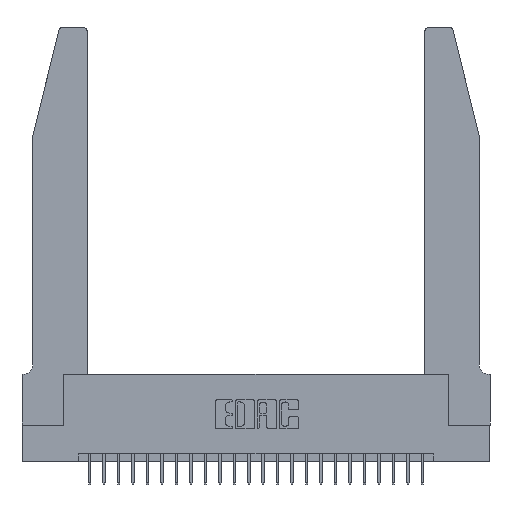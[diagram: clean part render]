
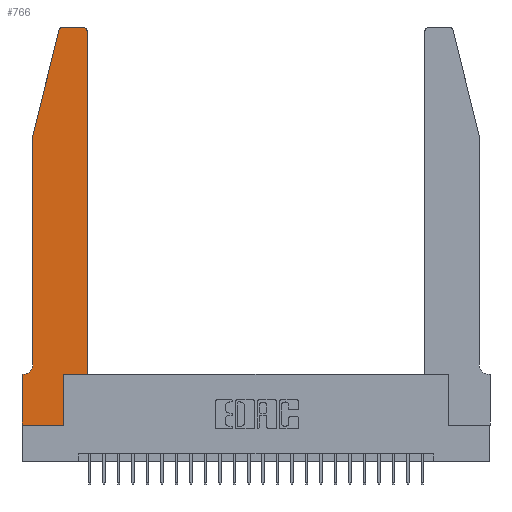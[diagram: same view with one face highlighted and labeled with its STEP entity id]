
A CAD part, top view. The second image highlights one B-rep face of the part: STEP entity #766.
In plain terms, the highlighted planar face has unit normal (0, 0, 1).
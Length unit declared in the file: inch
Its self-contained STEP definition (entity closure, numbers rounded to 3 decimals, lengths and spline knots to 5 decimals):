
#154 = CARTESIAN_POINT ( 'NONE',  ( 0.4505, 0.35, 0.37 ) ) ;
#517 = LINE ( 'NONE', #7419, #10268 ) ;
#766 = ADVANCED_FACE ( 'NONE', ( #21675 ), #9268, .T. ) ;
#827 = EDGE_CURVE ( 'NONE', #11715, #16014, #4376, .T. ) ;
#1599 = VERTEX_POINT ( 'NONE', #9152 ) ;
#2310 = DIRECTION ( 'NONE',  ( 0., 1., 0. ) ) ;
#3278 = EDGE_CURVE ( 'NONE', #14637, #11715, #20070, .T. ) ;
#4025 = CARTESIAN_POINT ( 'NONE',  ( 0., 0., 0.37 ) ) ;
#4050 = VECTOR ( 'NONE', #2310, 39.37008 ) ;
#4246 = ORIENTED_EDGE ( 'NONE', *, *, #5903, .T. ) ;
#4376 = LINE ( 'NONE', #4025, #19805 ) ;
#4411 = EDGE_CURVE ( 'NONE', #21281, #14637, #6228, .T. ) ;
#4421 = ORIENTED_EDGE ( 'NONE', *, *, #7641, .T. ) ;
#4755 = LINE ( 'NONE', #24394, #8960 ) ;
#4835 = CARTESIAN_POINT ( 'NONE',  ( 0.0055, 0.35, 0.37 ) ) ;
#4850 = CARTESIAN_POINT ( 'NONE',  ( 0.0755, 0.35, 0.37 ) ) ;
#4903 = VECTOR ( 'NONE', #20922, 39.37008 ) ;
#5070 = CARTESIAN_POINT ( 'NONE',  ( 0.0755, 2., 0.37 ) ) ;
#5484 = CARTESIAN_POINT ( 'NONE',  ( 0.2865, 0., 0.37 ) ) ;
#5593 = ORIENTED_EDGE ( 'NONE', *, *, #4411, .T. ) ;
#5618 = DIRECTION ( 'NONE',  ( 0., -1., 0. ) ) ;
#5797 = DIRECTION ( 'NONE',  ( 1., 0., 0. ) ) ;
#5903 = EDGE_CURVE ( 'NONE', #15294, #24518, #16241, .T. ) ;
#6228 = LINE ( 'NONE', #4850, #4903 ) ;
#6866 = LINE ( 'NONE', #19316, #15716 ) ;
#6924 = CARTESIAN_POINT ( 'NONE',  ( 0.2865, 0.35, 0.37 ) ) ;
#7098 = ORIENTED_EDGE ( 'NONE', *, *, #3278, .T. ) ;
#7419 = CARTESIAN_POINT ( 'NONE',  ( 0.2865, 0.35, 0.37 ) ) ;
#7463 = CARTESIAN_POINT ( 'NONE',  ( 0.2605, 2.75, 0.37 ) ) ;
#7641 = EDGE_CURVE ( 'NONE', #16014, #21268, #517, .T. ) ;
#7769 = VECTOR ( 'NONE', #21515, 39.37008 ) ;
#8455 = CARTESIAN_POINT ( 'NONE',  ( 0.0055, 0.42, 0.37 ) ) ;
#8582 = CARTESIAN_POINT ( 'NONE',  ( 0.4205, 2.72, 0.37 ) ) ;
#8960 = VECTOR ( 'NONE', #12621, 39.37008 ) ;
#9152 = CARTESIAN_POINT ( 'NONE',  ( 0.4205, 2.75, 0.37 ) ) ;
#9268 = PLANE ( 'NONE',  #25389 ) ;
#9486 = VECTOR ( 'NONE', #16763, 39.37008 ) ;
#9494 = ORIENTED_EDGE ( 'NONE', *, *, #16354, .T. ) ;
#9497 = CARTESIAN_POINT ( 'NONE',  ( 0., 0.35, 0.37 ) ) ;
#10060 = DIRECTION ( 'NONE',  ( 0., 0., 1. ) ) ;
#10237 = DIRECTION ( 'NONE',  ( 1., 0., 0. ) ) ;
#10268 = VECTOR ( 'NONE', #21390, 39.37008 ) ;
#10269 = DIRECTION ( 'NONE',  ( 0., 0., 1. ) ) ;
#10503 = DIRECTION ( 'NONE',  ( -1., 0., 0. ) ) ;
#10630 = DIRECTION ( 'NONE',  ( 1., 0., 0. ) ) ;
#10718 = VERTEX_POINT ( 'NONE', #14892 ) ;
#10878 = ORIENTED_EDGE ( 'NONE', *, *, #827, .T. ) ;
#11054 = EDGE_CURVE ( 'NONE', #11189, #21281, #24035, .T. ) ;
#11189 = VERTEX_POINT ( 'NONE', #24664 ) ;
#11715 = VERTEX_POINT ( 'NONE', #19064 ) ;
#12621 = DIRECTION ( 'NONE',  ( 1., 0., 0. ) ) ;
#13153 = LINE ( 'NONE', #7463, #7769 ) ;
#13290 = LINE ( 'NONE', #21462, #17932 ) ;
#13433 = ORIENTED_EDGE ( 'NONE', *, *, #21473, .T. ) ;
#14637 = VERTEX_POINT ( 'NONE', #9497 ) ;
#14892 = CARTESIAN_POINT ( 'NONE',  ( 0.4505, 0.35, 0.37 ) ) ;
#15294 = VERTEX_POINT ( 'NONE', #23229 ) ;
#15489 = LINE ( 'NONE', #154, #4050 ) ;
#15716 = VECTOR ( 'NONE', #21317, 39.37008 ) ;
#16014 = VERTEX_POINT ( 'NONE', #5484 ) ;
#16241 = CIRCLE ( 'NONE', #22013, 0.03 ) ;
#16354 = EDGE_CURVE ( 'NONE', #21268, #10718, #4755, .T. ) ;
#16763 = DIRECTION ( 'NONE',  ( 0., -1., 0. ) ) ;
#17114 = AXIS2_PLACEMENT_3D ( 'NONE', #8455, #22368, #10503 ) ;
#17373 = CIRCLE ( 'NONE', #18738, 0.03 ) ;
#17544 = ORIENTED_EDGE ( 'NONE', *, *, #23527, .T. ) ;
#17686 = ORIENTED_EDGE ( 'NONE', *, *, #18019, .T. ) ;
#17932 = VECTOR ( 'NONE', #5618, 39.37008 ) ;
#18019 = EDGE_CURVE ( 'NONE', #19070, #11189, #13290, .T. ) ;
#18260 = VERTEX_POINT ( 'NONE', #24596 ) ;
#18725 = CARTESIAN_POINT ( 'NONE',  ( 0., 0., 0.37 ) ) ;
#18738 = AXIS2_PLACEMENT_3D ( 'NONE', #8582, #22500, #10630 ) ;
#19064 = CARTESIAN_POINT ( 'NONE',  ( 0., 0., 0.37 ) ) ;
#19070 = VERTEX_POINT ( 'NONE', #5070 ) ;
#19238 = ORIENTED_EDGE ( 'NONE', *, *, #24124, .T. ) ;
#19316 = CARTESIAN_POINT ( 'NONE',  ( 0.0755, 2., 0.37 ) ) ;
#19805 = VECTOR ( 'NONE', #5797, 39.37008 ) ;
#20018 = EDGE_CURVE ( 'NONE', #24518, #19070, #6866, .T. ) ;
#20070 = LINE ( 'NONE', #18725, #9486 ) ;
#20133 = CARTESIAN_POINT ( 'NONE',  ( 0.25487, 2.72718, 0.37 ) ) ;
#20535 = ORIENTED_EDGE ( 'NONE', *, *, #20018, .T. ) ;
#20922 = DIRECTION ( 'NONE',  ( -1., 0., 0. ) ) ;
#21268 = VERTEX_POINT ( 'NONE', #6924 ) ;
#21281 = VERTEX_POINT ( 'NONE', #4835 ) ;
#21317 = DIRECTION ( 'NONE',  ( -0.239, -0.971, 0. ) ) ;
#21390 = DIRECTION ( 'NONE',  ( 0., 1., 0. ) ) ;
#21462 = CARTESIAN_POINT ( 'NONE',  ( 0.0755, 2., 0.37 ) ) ;
#21473 = EDGE_CURVE ( 'NONE', #1599, #15294, #13153, .T. ) ;
#21515 = DIRECTION ( 'NONE',  ( -1., 0., 0. ) ) ;
#21675 = FACE_OUTER_BOUND ( 'NONE', #21859, .T. ) ;
#21859 = EDGE_LOOP ( 'NONE', ( #13433, #4246, #20535, #17686, #21932, #5593, #7098, #10878, #4421, #9494, #19238, #17544 ) ) ;
#21932 = ORIENTED_EDGE ( 'NONE', *, *, #11054, .T. ) ;
#22013 = AXIS2_PLACEMENT_3D ( 'NONE', #22130, #10269, #24109 ) ;
#22130 = CARTESIAN_POINT ( 'NONE',  ( 0.284, 2.72, 0.37 ) ) ;
#22368 = DIRECTION ( 'NONE',  ( 0., 0., -1. ) ) ;
#22500 = DIRECTION ( 'NONE',  ( 0., 0., 1. ) ) ;
#23229 = CARTESIAN_POINT ( 'NONE',  ( 0.284, 2.75, 0.37 ) ) ;
#23527 = EDGE_CURVE ( 'NONE', #18260, #1599, #17373, .T. ) ;
#24035 = CIRCLE ( 'NONE', #17114, 0.07 ) ;
#24109 = DIRECTION ( 'NONE',  ( 1., 0., 0. ) ) ;
#24124 = EDGE_CURVE ( 'NONE', #10718, #18260, #15489, .T. ) ;
#24394 = CARTESIAN_POINT ( 'NONE',  ( 0.4505, 0.35, 0.37 ) ) ;
#24518 = VERTEX_POINT ( 'NONE', #20133 ) ;
#24596 = CARTESIAN_POINT ( 'NONE',  ( 0.4505, 2.72, 0.37 ) ) ;
#24664 = CARTESIAN_POINT ( 'NONE',  ( 0.0755, 0.42, 0.37 ) ) ;
#25389 = AXIS2_PLACEMENT_3D ( 'NONE', #25616, #10060, #10237 ) ;
#25616 = CARTESIAN_POINT ( 'NONE',  ( 0., 0.35, 0.37 ) ) ;
